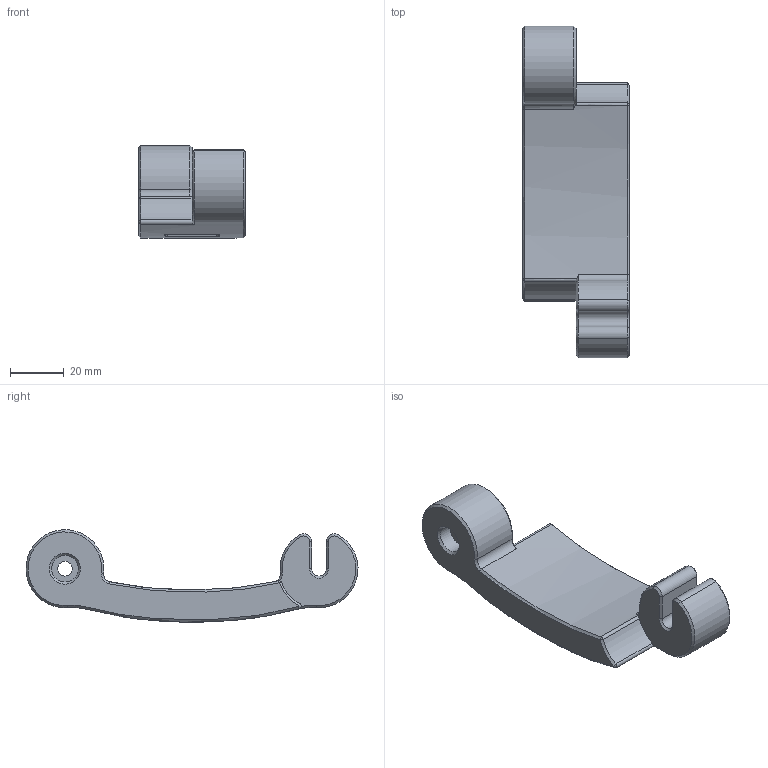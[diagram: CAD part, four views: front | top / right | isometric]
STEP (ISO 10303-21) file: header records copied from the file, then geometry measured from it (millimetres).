
FILE_DESCRIPTION (( 'STEP AP203' ), '1' );
FILE_NAME ('WTF-9_stock_brace_2.STEP', '2020-05-09T10:21:44', ( '' ), ( '' ), 'SwSTEP 2.0', 'SolidWorks 2016', '' );
FILE_SCHEMA (( 'CONFIG_CONTROL_DESIGN' ));
Length unit declared in the file: millimetre
Products named in the file (2): WTF9 V1 FINAL_14; WTF-9_stock_brace_2
Assembly tree (1 placements, depth 2):
  WTF-9_stock_brace_2
    WTF9 V1 FINAL_14
Bounding box: 40 x 124.12 x 34.55 mm (x, y, z)
Volume: 56777.3 mm3; surface area: 16249.8 mm2
Topology: 1 solids, 1 shells, 87 faces, 202 edges, 118 vertices
Faces by surface type: bspline 27, cone 23, cylinder 20, plane 13, torus 4
Full cylindrical faces by diameter (mm): 5.5 x1, 10 x1
Entity records: 3702 total; most frequent: CARTESIAN_POINT 1731, ORIENTED_EDGE 396, DIRECTION 316, EDGE_CURVE 198, AXIS2_PLACEMENT_3D 124, VERTEX_POINT 118, EDGE_LOOP 96, FACE_OUTER_BOUND 89
